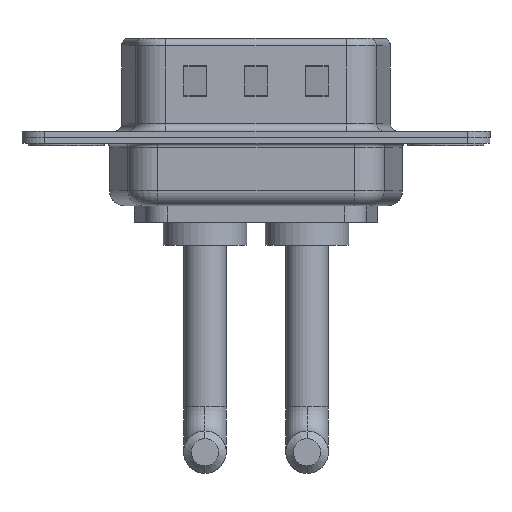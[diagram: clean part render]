
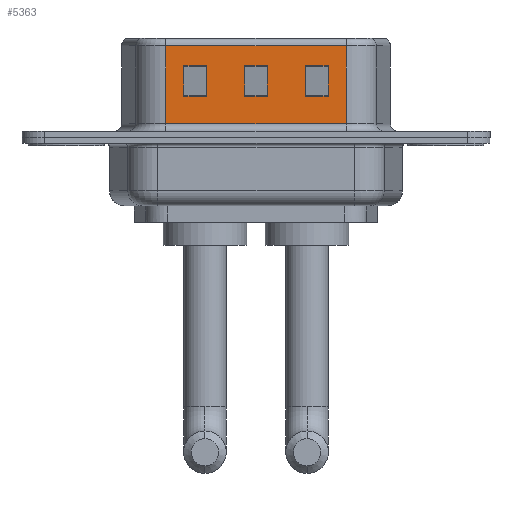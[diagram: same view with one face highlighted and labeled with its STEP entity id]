
A CAD part, front view. The second image highlights one B-rep face of the part: STEP entity #5363.
In plain terms, the highlighted planar face has unit normal (0, -1, 0).
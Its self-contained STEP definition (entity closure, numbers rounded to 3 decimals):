
#10 = LINE ( 'NONE', #10420, #3687 ) ;
#349 = CARTESIAN_POINT ( 'NONE',  ( 15.75, -4.55, 6.52 ) ) ;
#388 = DIRECTION ( 'NONE',  ( 0., 0., -1. ) ) ;
#513 = VECTOR ( 'NONE', #1330, 1000. ) ;
#561 = ORIENTED_EDGE ( 'NONE', *, *, #8463, .T. ) ;
#598 = ORIENTED_EDGE ( 'NONE', *, *, #5630, .T. ) ;
#625 = VECTOR ( 'NONE', #1133, 1000. ) ;
#699 = FACE_BOUND ( 'NONE', #3153, .T. ) ;
#726 = EDGE_CURVE ( 'NONE', #5534, #11903, #11821, .T. ) ;
#868 = ORIENTED_EDGE ( 'NONE', *, *, #10007, .T. ) ;
#891 = CARTESIAN_POINT ( 'NONE',  ( 13.25, -4.55, 2.705 ) ) ;
#990 = VERTEX_POINT ( 'NONE', #4960 ) ;
#1133 = DIRECTION ( 'NONE',  ( 1., 0., 0. ) ) ;
#1189 = CARTESIAN_POINT ( 'NONE',  ( 18.451, -4.55, 6.02 ) ) ;
#1330 = DIRECTION ( 'NONE',  ( 0., 0., -1. ) ) ;
#1368 = LINE ( 'NONE', #1189, #9669 ) ;
#1443 = LINE ( 'NONE', #6084, #8570 ) ;
#1480 = EDGE_CURVE ( 'NONE', #5127, #2692, #1368, .T. ) ;
#1719 = CARTESIAN_POINT ( 'NONE',  ( 18.451, -4.55, 4.705 ) ) ;
#1856 = DIRECTION ( 'NONE',  ( 1., 0., 0. ) ) ;
#1872 = DIRECTION ( 'NONE',  ( 0., 0., -1. ) ) ;
#1904 = DIRECTION ( 'NONE',  ( 1., 0., 0. ) ) ;
#1932 = LINE ( 'NONE', #3116, #6462 ) ;
#1949 = CARTESIAN_POINT ( 'NONE',  ( 11.75, -4.55, 4.705 ) ) ;
#2247 = CARTESIAN_POINT ( 'NONE',  ( 9.25, -4.55, 6.52 ) ) ;
#2403 = DIRECTION ( 'NONE',  ( 0., 0., 1. ) ) ;
#2454 = VECTOR ( 'NONE', #8496, 1000. ) ;
#2540 = DIRECTION ( 'NONE',  ( 0., 0., -1. ) ) ;
#2556 = DIRECTION ( 'NONE',  ( -1., 0., 0. ) ) ;
#2692 = VERTEX_POINT ( 'NONE', #10719 ) ;
#2809 = LINE ( 'NONE', #4715, #4894 ) ;
#2819 = CARTESIAN_POINT ( 'NONE',  ( 6.549, -4.55, 6.52 ) ) ;
#2899 = EDGE_CURVE ( 'NONE', #4064, #7279, #11853, .T. ) ;
#2974 = CARTESIAN_POINT ( 'NONE',  ( 17.25, -4.55, 2.705 ) ) ;
#3033 = EDGE_CURVE ( 'NONE', #11903, #10059, #5510, .T. ) ;
#3064 = VECTOR ( 'NONE', #2540, 1000. ) ;
#3075 = CARTESIAN_POINT ( 'NONE',  ( 11.75, -4.55, 2.705 ) ) ;
#3101 = EDGE_CURVE ( 'NONE', #5391, #4731, #7799, .T. ) ;
#3107 = ORIENTED_EDGE ( 'NONE', *, *, #2899, .T. ) ;
#3116 = CARTESIAN_POINT ( 'NONE',  ( 14.451, -4.55, 4.705 ) ) ;
#3134 = EDGE_CURVE ( 'NONE', #3298, #5099, #7673, .T. ) ;
#3153 = EDGE_LOOP ( 'NONE', ( #561, #12441, #8508, #11267 ) ) ;
#3298 = VERTEX_POINT ( 'NONE', #9102 ) ;
#3310 = EDGE_CURVE ( 'NONE', #8328, #3298, #8863, .T. ) ;
#3336 = CARTESIAN_POINT ( 'NONE',  ( 18.451, -4.55, 0.9 ) ) ;
#3625 = CARTESIAN_POINT ( 'NONE',  ( 9.25, -4.55, 4.705 ) ) ;
#3676 = CARTESIAN_POINT ( 'NONE',  ( 18.451, -4.55, 0.9 ) ) ;
#3687 = VECTOR ( 'NONE', #5799, 1000. ) ;
#3795 = FACE_OUTER_BOUND ( 'NONE', #6418, .T. ) ;
#3839 = EDGE_CURVE ( 'NONE', #10059, #4568, #1443, .T. ) ;
#3880 = VECTOR ( 'NONE', #4276, 1000. ) ;
#3994 = CARTESIAN_POINT ( 'NONE',  ( 18.451, -4.55, 6.02 ) ) ;
#4064 = VERTEX_POINT ( 'NONE', #5768 ) ;
#4276 = DIRECTION ( 'NONE',  ( 0., 0., 1. ) ) ;
#4286 = EDGE_LOOP ( 'NONE', ( #9166, #868, #12459, #11507 ) ) ;
#4548 = VERTEX_POINT ( 'NONE', #1949 ) ;
#4568 = VERTEX_POINT ( 'NONE', #5872 ) ;
#4575 = LINE ( 'NONE', #1719, #8293 ) ;
#4657 = VECTOR ( 'NONE', #2403, 1000. ) ;
#4715 = CARTESIAN_POINT ( 'NONE',  ( 22.451, -4.55, 2.705 ) ) ;
#4731 = VERTEX_POINT ( 'NONE', #3075 ) ;
#4767 = DIRECTION ( 'NONE',  ( -1., 0., 0. ) ) ;
#4894 = VECTOR ( 'NONE', #2556, 1000. ) ;
#4960 = CARTESIAN_POINT ( 'NONE',  ( 13.25, -4.55, 4.705 ) ) ;
#5055 = EDGE_CURVE ( 'NONE', #5099, #10977, #10, .T. ) ;
#5093 = DIRECTION ( 'NONE',  ( 1., 0., 0. ) ) ;
#5096 = VECTOR ( 'NONE', #7744, 1000. ) ;
#5099 = VERTEX_POINT ( 'NONE', #5146 ) ;
#5122 = EDGE_CURVE ( 'NONE', #990, #5391, #10979, .T. ) ;
#5127 = VERTEX_POINT ( 'NONE', #3994 ) ;
#5146 = CARTESIAN_POINT ( 'NONE',  ( 17.25, -4.55, 4.705 ) ) ;
#5279 = EDGE_LOOP ( 'NONE', ( #10017, #11253, #6711, #598 ) ) ;
#5363 = ADVANCED_FACE ( 'NONE', ( #12573, #5784, #699, #3795 ), #11548, .F. ) ;
#5391 = VERTEX_POINT ( 'NONE', #891 ) ;
#5448 = EDGE_CURVE ( 'NONE', #2692, #4064, #6622, .T. ) ;
#5510 = LINE ( 'NONE', #6459, #2454 ) ;
#5534 = VERTEX_POINT ( 'NONE', #3625 ) ;
#5630 = EDGE_CURVE ( 'NONE', #4568, #5534, #1932, .T. ) ;
#5768 = CARTESIAN_POINT ( 'NONE',  ( 6.549, -4.55, 0.9 ) ) ;
#5784 = FACE_BOUND ( 'NONE', #4286, .T. ) ;
#5799 = DIRECTION ( 'NONE',  ( 0., 0., -1. ) ) ;
#5826 = CARTESIAN_POINT ( 'NONE',  ( 18.451, -4.55, 2.705 ) ) ;
#5872 = CARTESIAN_POINT ( 'NONE',  ( 7.75, -4.55, 4.705 ) ) ;
#5917 = CARTESIAN_POINT ( 'NONE',  ( 13.25, -4.55, 6.52 ) ) ;
#6084 = CARTESIAN_POINT ( 'NONE',  ( 7.75, -4.55, 6.52 ) ) ;
#6418 = EDGE_LOOP ( 'NONE', ( #10381, #8234, #8141, #3107 ) ) ;
#6459 = CARTESIAN_POINT ( 'NONE',  ( 14.451, -4.55, 2.705 ) ) ;
#6462 = VECTOR ( 'NONE', #5093, 1000. ) ;
#6622 = LINE ( 'NONE', #2819, #9124 ) ;
#6711 = ORIENTED_EDGE ( 'NONE', *, *, #3839, .T. ) ;
#7224 = DIRECTION ( 'NONE',  ( 0., 0., 1. ) ) ;
#7279 = VERTEX_POINT ( 'NONE', #3676 ) ;
#7511 = CARTESIAN_POINT ( 'NONE',  ( 7.75, -4.55, 2.705 ) ) ;
#7673 = LINE ( 'NONE', #11533, #12188 ) ;
#7689 = DIRECTION ( 'NONE',  ( 0., 1., 0. ) ) ;
#7744 = DIRECTION ( 'NONE',  ( -1., 0., 0. ) ) ;
#7799 = LINE ( 'NONE', #5826, #5096 ) ;
#8141 = ORIENTED_EDGE ( 'NONE', *, *, #5448, .T. ) ;
#8234 = ORIENTED_EDGE ( 'NONE', *, *, #1480, .T. ) ;
#8293 = VECTOR ( 'NONE', #1856, 1000. ) ;
#8303 = LINE ( 'NONE', #12047, #4657 ) ;
#8328 = VERTEX_POINT ( 'NONE', #11165 ) ;
#8463 = EDGE_CURVE ( 'NONE', #4548, #990, #4575, .T. ) ;
#8496 = DIRECTION ( 'NONE',  ( -1., 0., 0. ) ) ;
#8508 = ORIENTED_EDGE ( 'NONE', *, *, #3101, .T. ) ;
#8570 = VECTOR ( 'NONE', #7224, 1000. ) ;
#8653 = CARTESIAN_POINT ( 'NONE',  ( 9.25, -4.55, 2.705 ) ) ;
#8855 = EDGE_CURVE ( 'NONE', #4731, #4548, #8303, .T. ) ;
#8863 = LINE ( 'NONE', #349, #3880 ) ;
#8936 = DIRECTION ( 'NONE',  ( -1., 0., 0. ) ) ;
#9102 = CARTESIAN_POINT ( 'NONE',  ( 15.75, -4.55, 4.705 ) ) ;
#9124 = VECTOR ( 'NONE', #1872, 1000. ) ;
#9166 = ORIENTED_EDGE ( 'NONE', *, *, #5055, .T. ) ;
#9390 = LINE ( 'NONE', #12382, #3064 ) ;
#9669 = VECTOR ( 'NONE', #8936, 1000. ) ;
#9734 = AXIS2_PLACEMENT_3D ( 'NONE', #12389, #7689, #4767 ) ;
#10007 = EDGE_CURVE ( 'NONE', #10977, #8328, #2809, .T. ) ;
#10017 = ORIENTED_EDGE ( 'NONE', *, *, #726, .T. ) ;
#10059 = VERTEX_POINT ( 'NONE', #7511 ) ;
#10381 = ORIENTED_EDGE ( 'NONE', *, *, #10471, .F. ) ;
#10420 = CARTESIAN_POINT ( 'NONE',  ( 17.25, -4.55, 6.52 ) ) ;
#10471 = EDGE_CURVE ( 'NONE', #5127, #7279, #9390, .T. ) ;
#10645 = VECTOR ( 'NONE', #388, 1000. ) ;
#10719 = CARTESIAN_POINT ( 'NONE',  ( 6.549, -4.55, 6.02 ) ) ;
#10977 = VERTEX_POINT ( 'NONE', #2974 ) ;
#10979 = LINE ( 'NONE', #5917, #513 ) ;
#11165 = CARTESIAN_POINT ( 'NONE',  ( 15.75, -4.55, 2.705 ) ) ;
#11253 = ORIENTED_EDGE ( 'NONE', *, *, #3033, .T. ) ;
#11267 = ORIENTED_EDGE ( 'NONE', *, *, #8855, .T. ) ;
#11507 = ORIENTED_EDGE ( 'NONE', *, *, #3134, .T. ) ;
#11533 = CARTESIAN_POINT ( 'NONE',  ( 22.451, -4.55, 4.705 ) ) ;
#11548 = PLANE ( 'NONE',  #9734 ) ;
#11821 = LINE ( 'NONE', #2247, #10645 ) ;
#11853 = LINE ( 'NONE', #3336, #625 ) ;
#11903 = VERTEX_POINT ( 'NONE', #8653 ) ;
#12047 = CARTESIAN_POINT ( 'NONE',  ( 11.75, -4.55, 6.52 ) ) ;
#12188 = VECTOR ( 'NONE', #1904, 1000. ) ;
#12382 = CARTESIAN_POINT ( 'NONE',  ( 18.451, -4.55, 6.52 ) ) ;
#12389 = CARTESIAN_POINT ( 'NONE',  ( 18.451, -4.55, 6.52 ) ) ;
#12441 = ORIENTED_EDGE ( 'NONE', *, *, #5122, .T. ) ;
#12459 = ORIENTED_EDGE ( 'NONE', *, *, #3310, .T. ) ;
#12573 = FACE_BOUND ( 'NONE', #5279, .T. ) ;
